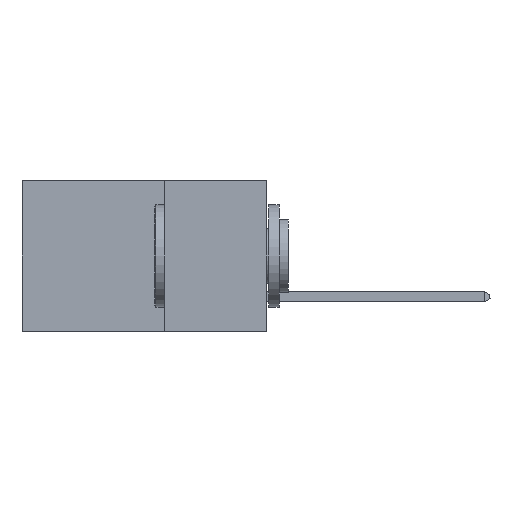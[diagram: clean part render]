
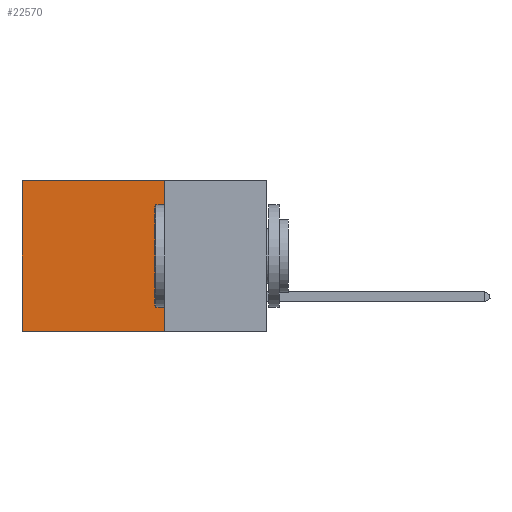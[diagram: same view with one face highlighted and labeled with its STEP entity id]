
A CAD part, left-side view. The second image highlights one B-rep face of the part: STEP entity #22570.
In plain terms, the highlighted planar face has unit normal (-1, 0, 0).
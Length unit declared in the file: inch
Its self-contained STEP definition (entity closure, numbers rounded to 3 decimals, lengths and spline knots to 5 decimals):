
#592 = CARTESIAN_POINT ( 'NONE',  ( 0.2875, 0.25, 0. ) ) ;
#3494 = DIRECTION ( 'NONE',  ( 0., 0., -1. ) ) ;
#4228 = LINE ( 'NONE', #9481, #14566 ) ;
#5527 = LINE ( 'NONE', #25141, #27561 ) ;
#5615 = DIRECTION ( 'NONE',  ( 0., 0., -1. ) ) ;
#6614 = CARTESIAN_POINT ( 'NONE',  ( 0.2875, 0.6, 0. ) ) ;
#7578 = CARTESIAN_POINT ( 'NONE',  ( 0.2875, 0.25, 0. ) ) ;
#7679 = VECTOR ( 'NONE', #3494, 39.37008 ) ;
#7853 = ORIENTED_EDGE ( 'NONE', *, *, #21771, .T. ) ;
#8330 = AXIS2_PLACEMENT_3D ( 'NONE', #7578, #18783, #27665 ) ;
#9058 = CARTESIAN_POINT ( 'NONE',  ( 0.2875, 0.25, -0.37 ) ) ;
#9481 = CARTESIAN_POINT ( 'NONE',  ( 0.2875, 0.25, 0. ) ) ;
#9582 = CARTESIAN_POINT ( 'NONE',  ( 0.2875, 0.25, 0. ) ) ;
#10836 = LINE ( 'NONE', #592, #7679 ) ;
#11231 = CARTESIAN_POINT ( 'NONE',  ( 0.2875, 0.25, -0.37 ) ) ;
#11614 = FACE_OUTER_BOUND ( 'NONE', #31423, .T. ) ;
#11962 = DIRECTION ( 'NONE',  ( 0., 1., 0. ) ) ;
#14217 = VERTEX_POINT ( 'NONE', #11231 ) ;
#14566 = VECTOR ( 'NONE', #18421, 39.37008 ) ;
#14827 = VERTEX_POINT ( 'NONE', #9582 ) ;
#16086 = LINE ( 'NONE', #9058, #25144 ) ;
#18321 = EDGE_CURVE ( 'NONE', #14217, #26402, #16086, .T. ) ;
#18421 = DIRECTION ( 'NONE',  ( 0., 1., 0. ) ) ;
#18783 = DIRECTION ( 'NONE',  ( 1., 0., 0. ) ) ;
#21303 = ORIENTED_EDGE ( 'NONE', *, *, #18321, .F. ) ;
#21771 = EDGE_CURVE ( 'NONE', #28470, #26402, #5527, .T. ) ;
#22570 = ADVANCED_FACE ( 'NONE', ( #11614 ), #24800, .F. ) ;
#24299 = EDGE_CURVE ( 'NONE', #14827, #28470, #4228, .T. ) ;
#24800 = PLANE ( 'NONE',  #8330 ) ;
#25141 = CARTESIAN_POINT ( 'NONE',  ( 0.2875, 0.6, 0. ) ) ;
#25144 = VECTOR ( 'NONE', #11962, 39.37008 ) ;
#26402 = VERTEX_POINT ( 'NONE', #28716 ) ;
#27492 = EDGE_CURVE ( 'NONE', #14827, #14217, #10836, .T. ) ;
#27561 = VECTOR ( 'NONE', #5615, 39.37008 ) ;
#27665 = DIRECTION ( 'NONE',  ( 0., 0., -1. ) ) ;
#28470 = VERTEX_POINT ( 'NONE', #6614 ) ;
#28716 = CARTESIAN_POINT ( 'NONE',  ( 0.2875, 0.6, -0.37 ) ) ;
#29625 = ORIENTED_EDGE ( 'NONE', *, *, #27492, .F. ) ;
#31423 = EDGE_LOOP ( 'NONE', ( #7853, #21303, #29625, #35031 ) ) ;
#35031 = ORIENTED_EDGE ( 'NONE', *, *, #24299, .T. ) ;
